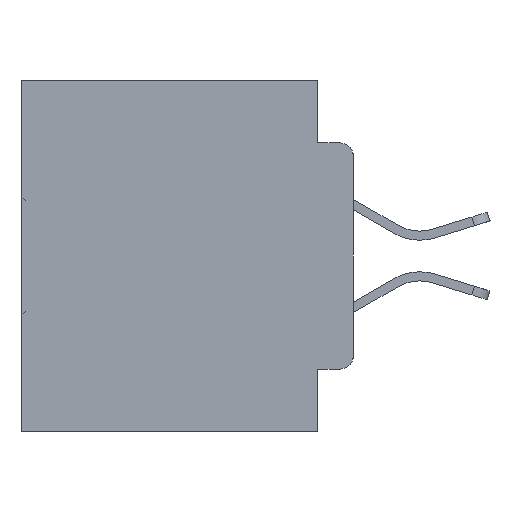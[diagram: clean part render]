
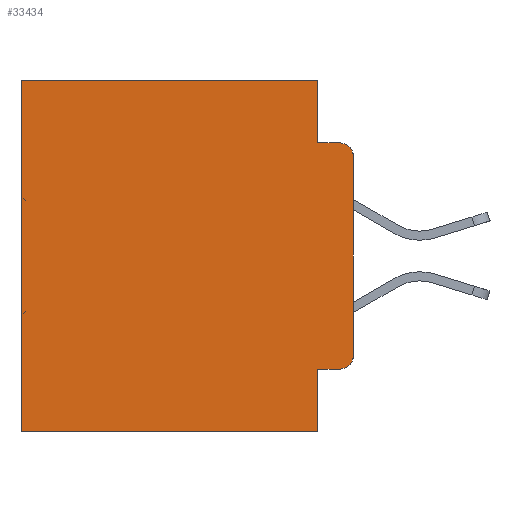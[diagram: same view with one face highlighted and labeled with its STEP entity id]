
A CAD part, left-side view. The second image highlights one B-rep face of the part: STEP entity #33434.
In plain terms, the highlighted planar face has unit normal (-1, 0, 0).
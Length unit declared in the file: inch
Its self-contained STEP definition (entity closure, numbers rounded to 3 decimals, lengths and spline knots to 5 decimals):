
#67 = CARTESIAN_POINT ( 'NONE',  ( 0.298, 0., -0.5 ) ) ;
#743 = LINE ( 'NONE', #3338, #30856 ) ;
#1339 = VECTOR ( 'NONE', #22387, 39.37008 ) ;
#1580 = ORIENTED_EDGE ( 'NONE', *, *, #7016, .F. ) ;
#2215 = VERTEX_POINT ( 'NONE', #9766 ) ;
#2913 = VERTEX_POINT ( 'NONE', #9297 ) ;
#3090 = CARTESIAN_POINT ( 'NONE',  ( 0.298, 0.051, -0.4115 ) ) ;
#3338 = CARTESIAN_POINT ( 'NONE',  ( 0.298, 0.051, 0. ) ) ;
#3500 = ORIENTED_EDGE ( 'NONE', *, *, #22186, .T. ) ;
#3534 = VECTOR ( 'NONE', #17964, 39.37008 ) ;
#3910 = DIRECTION ( 'NONE',  ( -1., 0., 0. ) ) ;
#3961 = CARTESIAN_POINT ( 'NONE',  ( 0.298, 0.473, 0. ) ) ;
#4912 = AXIS2_PLACEMENT_3D ( 'NONE', #7649, #10583, #18200 ) ;
#5459 = VERTEX_POINT ( 'NONE', #24564 ) ;
#5618 = VECTOR ( 'NONE', #8041, 39.37008 ) ;
#6504 = CARTESIAN_POINT ( 'NONE',  ( 0.298, 0.051, -0.0885 ) ) ;
#7016 = EDGE_CURVE ( 'NONE', #2913, #2215, #18290, .T. ) ;
#7057 = EDGE_CURVE ( 'NONE', #30786, #2215, #24521, .T. ) ;
#7649 = CARTESIAN_POINT ( 'NONE',  ( 0.298, 0.02, -0.3915 ) ) ;
#7880 = VERTEX_POINT ( 'NONE', #27449 ) ;
#7945 = LINE ( 'NONE', #3090, #27990 ) ;
#8041 = DIRECTION ( 'NONE',  ( 0., 1., 0. ) ) ;
#9198 = EDGE_CURVE ( 'NONE', #7880, #2913, #19044, .T. ) ;
#9297 = CARTESIAN_POINT ( 'NONE',  ( 0.298, 0.051, -0.0885 ) ) ;
#9668 = CARTESIAN_POINT ( 'NONE',  ( 0.298, 0.473, -0.5 ) ) ;
#9677 = LINE ( 'NONE', #33343, #33613 ) ;
#9766 = CARTESIAN_POINT ( 'NONE',  ( 0.298, 0.02, -0.0885 ) ) ;
#10397 = CARTESIAN_POINT ( 'NONE',  ( 0.298, 0., 0. ) ) ;
#10466 = ORIENTED_EDGE ( 'NONE', *, *, #11056, .F. ) ;
#10568 = FACE_OUTER_BOUND ( 'NONE', #30445, .T. ) ;
#10583 = DIRECTION ( 'NONE',  ( -1., 0., 0. ) ) ;
#10627 = DIRECTION ( 'NONE',  ( 0., 1., 0. ) ) ;
#10771 = ORIENTED_EDGE ( 'NONE', *, *, #11681, .F. ) ;
#11056 = EDGE_CURVE ( 'NONE', #29895, #21940, #23746, .T. ) ;
#11312 = CARTESIAN_POINT ( 'NONE',  ( 0.298, 0., 0. ) ) ;
#11355 = DIRECTION ( 'NONE',  ( 0., 0., -1. ) ) ;
#11475 = EDGE_CURVE ( 'NONE', #5459, #16562, #23105, .T. ) ;
#11681 = EDGE_CURVE ( 'NONE', #30786, #16562, #9677, .T. ) ;
#11944 = CARTESIAN_POINT ( 'NONE',  ( 0.298, 0., -0.3915 ) ) ;
#12411 = CARTESIAN_POINT ( 'NONE',  ( 0.298, 0.473, 0. ) ) ;
#12934 = AXIS2_PLACEMENT_3D ( 'NONE', #19126, #3910, #11355 ) ;
#14603 = CARTESIAN_POINT ( 'NONE',  ( 0.298, 0., -0.1085 ) ) ;
#14631 = EDGE_CURVE ( 'NONE', #7880, #18350, #18920, .T. ) ;
#15421 = DIRECTION ( 'NONE',  ( 1., 0., 0. ) ) ;
#16562 = VERTEX_POINT ( 'NONE', #11944 ) ;
#17110 = EDGE_CURVE ( 'NONE', #18350, #21940, #33489, .T. ) ;
#17964 = DIRECTION ( 'NONE',  ( 0., 0., -1. ) ) ;
#18200 = DIRECTION ( 'NONE',  ( 0., 0., -1. ) ) ;
#18205 = ORIENTED_EDGE ( 'NONE', *, *, #9198, .F. ) ;
#18290 = LINE ( 'NONE', #6504, #1339 ) ;
#18350 = VERTEX_POINT ( 'NONE', #3961 ) ;
#18911 = VERTEX_POINT ( 'NONE', #33711 ) ;
#18920 = LINE ( 'NONE', #11312, #5618 ) ;
#18991 = DIRECTION ( 'NONE',  ( 0., -1., 0. ) ) ;
#19044 = LINE ( 'NONE', #27786, #22976 ) ;
#19074 = DIRECTION ( 'NONE',  ( 0., 0., -1. ) ) ;
#19126 = CARTESIAN_POINT ( 'NONE',  ( 0.298, 0.02, -0.1085 ) ) ;
#21102 = PLANE ( 'NONE',  #33650 ) ;
#21135 = ORIENTED_EDGE ( 'NONE', *, *, #17110, .T. ) ;
#21357 = ORIENTED_EDGE ( 'NONE', *, *, #14631, .T. ) ;
#21940 = VERTEX_POINT ( 'NONE', #9668 ) ;
#21994 = VECTOR ( 'NONE', #10627, 39.37008 ) ;
#22186 = EDGE_CURVE ( 'NONE', #18911, #5459, #7945, .T. ) ;
#22387 = DIRECTION ( 'NONE',  ( 0., -1., 0. ) ) ;
#22975 = DIRECTION ( 'NONE',  ( 0., 0., -1. ) ) ;
#22976 = VECTOR ( 'NONE', #29918, 39.37008 ) ;
#23105 = CIRCLE ( 'NONE', #4912, 0.02 ) ;
#23746 = LINE ( 'NONE', #67, #21994 ) ;
#24521 = CIRCLE ( 'NONE', #12934, 0.02 ) ;
#24564 = CARTESIAN_POINT ( 'NONE',  ( 0.298, 0.02, -0.4115 ) ) ;
#25455 = EDGE_CURVE ( 'NONE', #18911, #29895, #743, .T. ) ;
#25602 = CARTESIAN_POINT ( 'NONE',  ( 0.298, 0.051, -0.5 ) ) ;
#27449 = CARTESIAN_POINT ( 'NONE',  ( 0.298, 0.051, 0. ) ) ;
#27786 = CARTESIAN_POINT ( 'NONE',  ( 0.298, 0.051, 0. ) ) ;
#27820 = ORIENTED_EDGE ( 'NONE', *, *, #25455, .F. ) ;
#27990 = VECTOR ( 'NONE', #18991, 39.37008 ) ;
#29772 = ORIENTED_EDGE ( 'NONE', *, *, #7057, .T. ) ;
#29895 = VERTEX_POINT ( 'NONE', #25602 ) ;
#29918 = DIRECTION ( 'NONE',  ( 0., 0., -1. ) ) ;
#30445 = EDGE_LOOP ( 'NONE', ( #10771, #29772, #1580, #18205, #21357, #21135, #10466, #27820, #3500, #30466 ) ) ;
#30466 = ORIENTED_EDGE ( 'NONE', *, *, #11475, .T. ) ;
#30786 = VERTEX_POINT ( 'NONE', #14603 ) ;
#30856 = VECTOR ( 'NONE', #19074, 39.37008 ) ;
#31813 = DIRECTION ( 'NONE',  ( 0., 0., -1. ) ) ;
#33343 = CARTESIAN_POINT ( 'NONE',  ( 0.298, 0., 0. ) ) ;
#33434 = ADVANCED_FACE ( 'NONE', ( #10568 ), #21102, .F. ) ;
#33489 = LINE ( 'NONE', #12411, #3534 ) ;
#33613 = VECTOR ( 'NONE', #22975, 39.37008 ) ;
#33650 = AXIS2_PLACEMENT_3D ( 'NONE', #10397, #15421, #31813 ) ;
#33711 = CARTESIAN_POINT ( 'NONE',  ( 0.298, 0.051, -0.4115 ) ) ;
